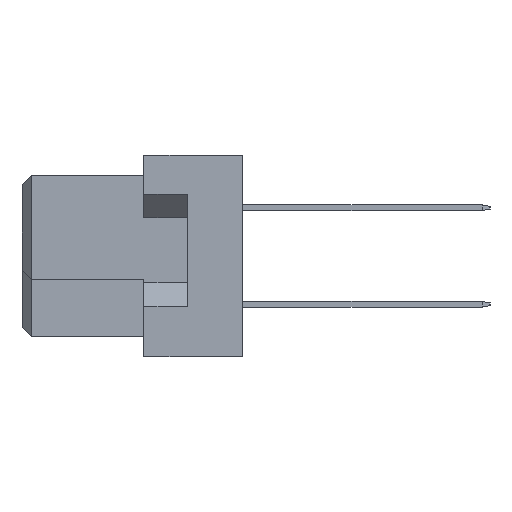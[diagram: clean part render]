
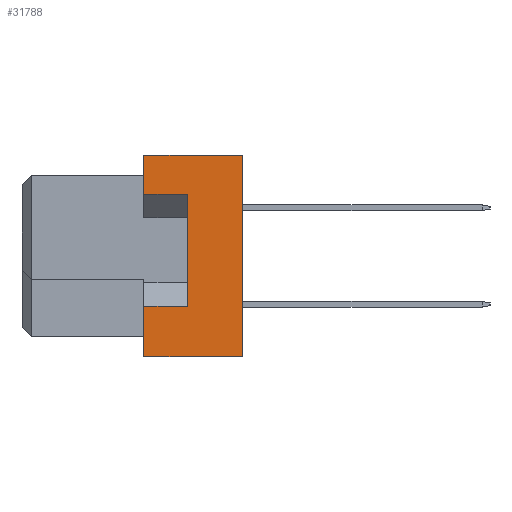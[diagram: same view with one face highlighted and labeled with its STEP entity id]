
A CAD part, left-side view. The second image highlights one B-rep face of the part: STEP entity #31788.
In plain terms, the highlighted planar face has unit normal (-1, 0, 0).
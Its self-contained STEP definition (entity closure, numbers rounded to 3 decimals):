
#2 = VERTEX_POINT ( 'NONE', #10916 ) ;
#2133 = LINE ( 'NONE', #11004, #20105 ) ;
#3260 = VERTEX_POINT ( 'NONE', #25923 ) ;
#3730 = CARTESIAN_POINT ( 'NONE',  ( -47.5, -8.7, -2.65 ) ) ;
#5775 = ORIENTED_EDGE ( 'NONE', *, *, #22203, .F. ) ;
#6007 = VERTEX_POINT ( 'NONE', #25323 ) ;
#6291 = CARTESIAN_POINT ( 'NONE',  ( -47.5, -8.7, -2.65 ) ) ;
#8106 = EDGE_CURVE ( 'NONE', #29495, #2, #33628, .T. ) ;
#8310 = LINE ( 'NONE', #14376, #34300 ) ;
#9031 = LINE ( 'NONE', #12655, #9692 ) ;
#9494 = EDGE_LOOP ( 'NONE', ( #20817, #27305, #17117, #35886, #11210, #32465, #35370, #5775 ) ) ;
#9692 = VECTOR ( 'NONE', #27355, 1000. ) ;
#10916 = CARTESIAN_POINT ( 'NONE',  ( -47.5, -6.4, 5.3 ) ) ;
#11004 = CARTESIAN_POINT ( 'NONE',  ( -47.5, -8.7, -2.65 ) ) ;
#11210 = ORIENTED_EDGE ( 'NONE', *, *, #22558, .T. ) ;
#11409 = DIRECTION ( 'NONE',  ( 0., 0., 1. ) ) ;
#11426 = VECTOR ( 'NONE', #14306, 1000. ) ;
#11799 = VECTOR ( 'NONE', #12297, 1000. ) ;
#12297 = DIRECTION ( 'NONE',  ( 0., 0., 1. ) ) ;
#12553 = DIRECTION ( 'NONE',  ( 0., 0., 1. ) ) ;
#12655 = CARTESIAN_POINT ( 'NONE',  ( -47.5, -11.6, -5.3 ) ) ;
#14306 = DIRECTION ( 'NONE',  ( 0., 1., 0. ) ) ;
#14376 = CARTESIAN_POINT ( 'NONE',  ( -47.5, -11.6, 5.3 ) ) ;
#14512 = EDGE_CURVE ( 'NONE', #6007, #16476, #32543, .T. ) ;
#15365 = DIRECTION ( 'NONE',  ( 0., 1., 0. ) ) ;
#16476 = VERTEX_POINT ( 'NONE', #19393 ) ;
#17116 = CARTESIAN_POINT ( 'NONE',  ( -47.5, -8.7, 3.25 ) ) ;
#17117 = ORIENTED_EDGE ( 'NONE', *, *, #32632, .F. ) ;
#19393 = CARTESIAN_POINT ( 'NONE',  ( -47.5, -11.6, 5.3 ) ) ;
#19912 = CARTESIAN_POINT ( 'NONE',  ( -47.5, -8.7, 3.25 ) ) ;
#20105 = VECTOR ( 'NONE', #11409, 1000. ) ;
#20817 = ORIENTED_EDGE ( 'NONE', *, *, #24080, .T. ) ;
#20832 = CARTESIAN_POINT ( 'NONE',  ( -47.5, -6.4, -2.65 ) ) ;
#21415 = FACE_OUTER_BOUND ( 'NONE', #9494, .T. ) ;
#21654 = VERTEX_POINT ( 'NONE', #20832 ) ;
#22203 = EDGE_CURVE ( 'NONE', #22479, #33934, #2133, .T. ) ;
#22479 = VERTEX_POINT ( 'NONE', #3730 ) ;
#22558 = EDGE_CURVE ( 'NONE', #16476, #2, #8310, .T. ) ;
#23530 = DIRECTION ( 'NONE',  ( 0., 0., 1. ) ) ;
#24080 = EDGE_CURVE ( 'NONE', #22479, #21654, #30664, .T. ) ;
#25323 = CARTESIAN_POINT ( 'NONE',  ( -47.5, -11.6, -5.3 ) ) ;
#25923 = CARTESIAN_POINT ( 'NONE',  ( -47.5, -6.4, -5.3 ) ) ;
#26712 = DIRECTION ( 'NONE',  ( 0., 0., 1. ) ) ;
#27291 = EDGE_CURVE ( 'NONE', #33934, #29495, #32416, .T. ) ;
#27305 = ORIENTED_EDGE ( 'NONE', *, *, #28865, .F. ) ;
#27355 = DIRECTION ( 'NONE',  ( 0., 1., 0. ) ) ;
#28865 = EDGE_CURVE ( 'NONE', #3260, #21654, #35187, .T. ) ;
#29055 = DIRECTION ( 'NONE',  ( 0., 1., 0. ) ) ;
#29495 = VERTEX_POINT ( 'NONE', #37885 ) ;
#30419 = CARTESIAN_POINT ( 'NONE',  ( -47.5, -6.4, -5.3 ) ) ;
#30659 = CARTESIAN_POINT ( 'NONE',  ( -47.5, -11.6, 5.3 ) ) ;
#30664 = LINE ( 'NONE', #6291, #34977 ) ;
#31267 = DIRECTION ( 'NONE',  ( -1., 0., 0. ) ) ;
#31788 = ADVANCED_FACE ( 'NONE', ( #21415 ), #36688, .T. ) ;
#32373 = CARTESIAN_POINT ( 'NONE',  ( -47.5, -6.4, -5.3 ) ) ;
#32416 = LINE ( 'NONE', #17116, #11426 ) ;
#32465 = ORIENTED_EDGE ( 'NONE', *, *, #8106, .F. ) ;
#32543 = LINE ( 'NONE', #35160, #34598 ) ;
#32632 = EDGE_CURVE ( 'NONE', #6007, #3260, #9031, .T. ) ;
#33628 = LINE ( 'NONE', #30419, #11799 ) ;
#33934 = VERTEX_POINT ( 'NONE', #19912 ) ;
#34300 = VECTOR ( 'NONE', #29055, 1000. ) ;
#34598 = VECTOR ( 'NONE', #26712, 1000. ) ;
#34977 = VECTOR ( 'NONE', #15365, 1000. ) ;
#35160 = CARTESIAN_POINT ( 'NONE',  ( -47.5, -11.6, 5.3 ) ) ;
#35187 = LINE ( 'NONE', #32373, #38488 ) ;
#35370 = ORIENTED_EDGE ( 'NONE', *, *, #27291, .F. ) ;
#35886 = ORIENTED_EDGE ( 'NONE', *, *, #14512, .T. ) ;
#36688 = PLANE ( 'NONE',  #37906 ) ;
#37885 = CARTESIAN_POINT ( 'NONE',  ( -47.5, -6.4, 3.25 ) ) ;
#37906 = AXIS2_PLACEMENT_3D ( 'NONE', #30659, #31267, #12553 ) ;
#38488 = VECTOR ( 'NONE', #23530, 1000. ) ;
